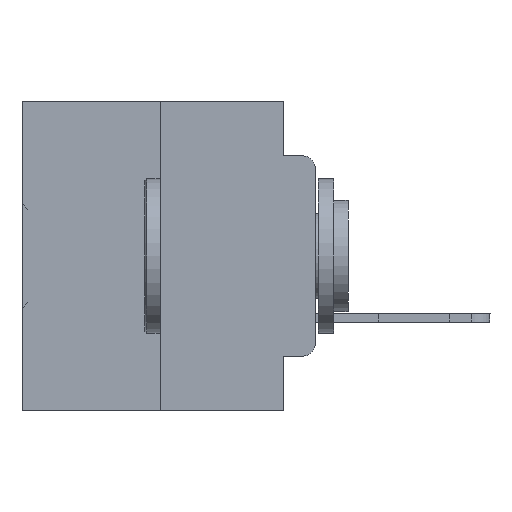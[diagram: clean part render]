
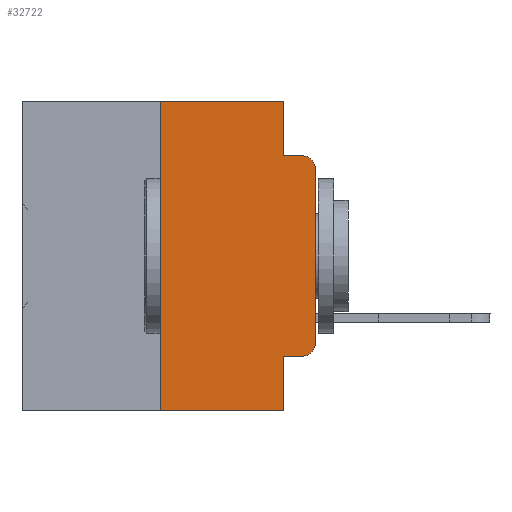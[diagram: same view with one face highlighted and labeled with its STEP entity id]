
A CAD part, left-side view. The second image highlights one B-rep face of the part: STEP entity #32722.
In plain terms, the highlighted planar face has unit normal (-1, 0, 0).
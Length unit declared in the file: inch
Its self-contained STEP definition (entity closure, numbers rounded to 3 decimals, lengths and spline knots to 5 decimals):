
#673 = ORIENTED_EDGE ( 'NONE', *, *, #14035, .F. ) ;
#1453 = ORIENTED_EDGE ( 'NONE', *, *, #7262, .T. ) ;
#1562 = LINE ( 'NONE', #12560, #15262 ) ;
#1902 = DIRECTION ( 'NONE',  ( -1., 0., 0. ) ) ;
#2042 = VERTEX_POINT ( 'NONE', #15241 ) ;
#2110 = CARTESIAN_POINT ( 'NONE',  ( 0., 0.473, 0. ) ) ;
#2149 = ORIENTED_EDGE ( 'NONE', *, *, #24073, .T. ) ;
#2264 = EDGE_CURVE ( 'NONE', #8409, #19866, #16018, .T. ) ;
#2404 = VERTEX_POINT ( 'NONE', #11795 ) ;
#2712 = CARTESIAN_POINT ( 'NONE',  ( 0., 0.25, 0. ) ) ;
#2730 = EDGE_CURVE ( 'NONE', #20173, #17940, #18801, .T. ) ;
#3554 = ORIENTED_EDGE ( 'NONE', *, *, #35037, .F. ) ;
#3657 = ORIENTED_EDGE ( 'NONE', *, *, #14612, .F. ) ;
#4195 = VECTOR ( 'NONE', #18595, 39.37008 ) ;
#4706 = LINE ( 'NONE', #10295, #4195 ) ;
#4924 = CARTESIAN_POINT ( 'NONE',  ( 0., 0.051, 0. ) ) ;
#5969 = LINE ( 'NONE', #19852, #33115 ) ;
#6812 = ORIENTED_EDGE ( 'NONE', *, *, #33802, .F. ) ;
#7262 = EDGE_CURVE ( 'NONE', #19866, #7368, #5969, .T. ) ;
#7368 = VERTEX_POINT ( 'NONE', #24902 ) ;
#7712 = VECTOR ( 'NONE', #22240, 39.37008 ) ;
#8409 = VERTEX_POINT ( 'NONE', #8639 ) ;
#8639 = CARTESIAN_POINT ( 'NONE',  ( 0., 0.02, -0.4115 ) ) ;
#10295 = CARTESIAN_POINT ( 'NONE',  ( 0., 0.051, -0.4115 ) ) ;
#10681 = CARTESIAN_POINT ( 'NONE',  ( 0., 0.473, 0. ) ) ;
#11225 = LINE ( 'NONE', #25462, #7712 ) ;
#11769 = CARTESIAN_POINT ( 'NONE',  ( 0., 0., -0.3915 ) ) ;
#11795 = CARTESIAN_POINT ( 'NONE',  ( 0., 0.051, -0.4115 ) ) ;
#12138 = CARTESIAN_POINT ( 'NONE',  ( 0., 0.25, -0.5 ) ) ;
#12560 = CARTESIAN_POINT ( 'NONE',  ( 0., 0.051, -0.0885 ) ) ;
#12630 = CARTESIAN_POINT ( 'NONE',  ( 0., 0.051, 0. ) ) ;
#12722 = CARTESIAN_POINT ( 'NONE',  ( 0., 0.02, -0.1085 ) ) ;
#13581 = DIRECTION ( 'NONE',  ( 0., 0., -1. ) ) ;
#14035 = EDGE_CURVE ( 'NONE', #22500, #20173, #15476, .T. ) ;
#14062 = DIRECTION ( 'NONE',  ( 0., 0., 1. ) ) ;
#14612 = EDGE_CURVE ( 'NONE', #27428, #21396, #1562, .T. ) ;
#14731 = ORIENTED_EDGE ( 'NONE', *, *, #18821, .T. ) ;
#15241 = CARTESIAN_POINT ( 'NONE',  ( 0., 0.051, -0.5 ) ) ;
#15262 = VECTOR ( 'NONE', #23575, 39.37008 ) ;
#15447 = CIRCLE ( 'NONE', #28709, 0.02 ) ;
#15476 = LINE ( 'NONE', #26477, #17562 ) ;
#15802 = VECTOR ( 'NONE', #20768, 39.37008 ) ;
#16018 = CIRCLE ( 'NONE', #27562, 0.02 ) ;
#17159 = CARTESIAN_POINT ( 'NONE',  ( 0., 0.051, -0.0885 ) ) ;
#17243 = EDGE_LOOP ( 'NONE', ( #1453, #34763, #3657, #3554, #18898, #673, #14731, #6812, #2149, #30284 ) ) ;
#17562 = VECTOR ( 'NONE', #34380, 39.37008 ) ;
#17940 = VERTEX_POINT ( 'NONE', #4924 ) ;
#18595 = DIRECTION ( 'NONE',  ( 0., -1., 0. ) ) ;
#18606 = CARTESIAN_POINT ( 'NONE',  ( 0., 0.02, -0.0885 ) ) ;
#18801 = LINE ( 'NONE', #10681, #21411 ) ;
#18821 = EDGE_CURVE ( 'NONE', #22500, #2042, #32228, .T. ) ;
#18898 = ORIENTED_EDGE ( 'NONE', *, *, #2730, .F. ) ;
#19251 = EDGE_CURVE ( 'NONE', #7368, #21396, #15447, .T. ) ;
#19429 = DIRECTION ( 'NONE',  ( 0., 0., -1. ) ) ;
#19738 = DIRECTION ( 'NONE',  ( -1., 0., 0. ) ) ;
#19852 = CARTESIAN_POINT ( 'NONE',  ( 0., 0., 0. ) ) ;
#19866 = VERTEX_POINT ( 'NONE', #11769 ) ;
#20173 = VERTEX_POINT ( 'NONE', #2712 ) ;
#20768 = DIRECTION ( 'NONE',  ( 0., 0., -1. ) ) ;
#20948 = LINE ( 'NONE', #12630, #15802 ) ;
#21396 = VERTEX_POINT ( 'NONE', #18606 ) ;
#21411 = VECTOR ( 'NONE', #35325, 39.37008 ) ;
#22240 = DIRECTION ( 'NONE',  ( 0., 0., -1. ) ) ;
#22448 = CARTESIAN_POINT ( 'NONE',  ( 0., 0.02, -0.3915 ) ) ;
#22500 = VERTEX_POINT ( 'NONE', #12138 ) ;
#23575 = DIRECTION ( 'NONE',  ( 0., -1., 0. ) ) ;
#23608 = CARTESIAN_POINT ( 'NONE',  ( 0., 0.473, -0.5 ) ) ;
#24073 = EDGE_CURVE ( 'NONE', #2404, #8409, #4706, .T. ) ;
#24902 = CARTESIAN_POINT ( 'NONE',  ( 0., 0., -0.1085 ) ) ;
#25462 = CARTESIAN_POINT ( 'NONE',  ( 0., 0.051, 0. ) ) ;
#25807 = VECTOR ( 'NONE', #26836, 39.37008 ) ;
#26477 = CARTESIAN_POINT ( 'NONE',  ( 0., 0.25, 0. ) ) ;
#26836 = DIRECTION ( 'NONE',  ( 0., -1., 0. ) ) ;
#27428 = VERTEX_POINT ( 'NONE', #17159 ) ;
#27562 = AXIS2_PLACEMENT_3D ( 'NONE', #22448, #19738, #13581 ) ;
#28709 = AXIS2_PLACEMENT_3D ( 'NONE', #12722, #1902, #28954 ) ;
#28954 = DIRECTION ( 'NONE',  ( 0., 0., -1. ) ) ;
#30051 = DIRECTION ( 'NONE',  ( 1., 0., 0. ) ) ;
#30284 = ORIENTED_EDGE ( 'NONE', *, *, #2264, .T. ) ;
#32228 = LINE ( 'NONE', #23608, #25807 ) ;
#32722 = ADVANCED_FACE ( 'NONE', ( #35416 ), #35056, .F. ) ;
#33115 = VECTOR ( 'NONE', #14062, 39.37008 ) ;
#33802 = EDGE_CURVE ( 'NONE', #2404, #2042, #20948, .T. ) ;
#34380 = DIRECTION ( 'NONE',  ( 0., 0., 1. ) ) ;
#34678 = AXIS2_PLACEMENT_3D ( 'NONE', #2110, #30051, #19429 ) ;
#34763 = ORIENTED_EDGE ( 'NONE', *, *, #19251, .T. ) ;
#35037 = EDGE_CURVE ( 'NONE', #17940, #27428, #11225, .T. ) ;
#35056 = PLANE ( 'NONE',  #34678 ) ;
#35325 = DIRECTION ( 'NONE',  ( 0., -1., 0. ) ) ;
#35416 = FACE_OUTER_BOUND ( 'NONE', #17243, .T. ) ;
